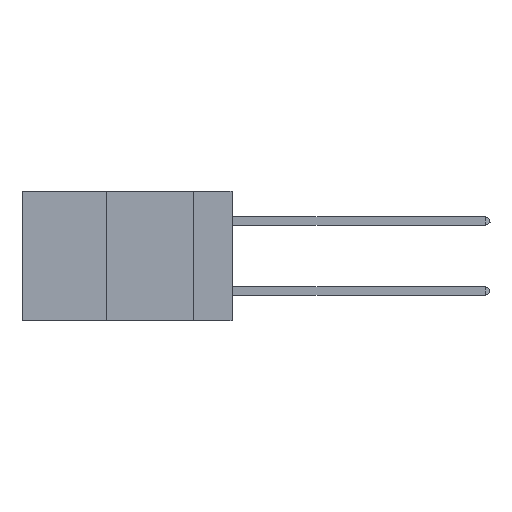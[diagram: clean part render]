
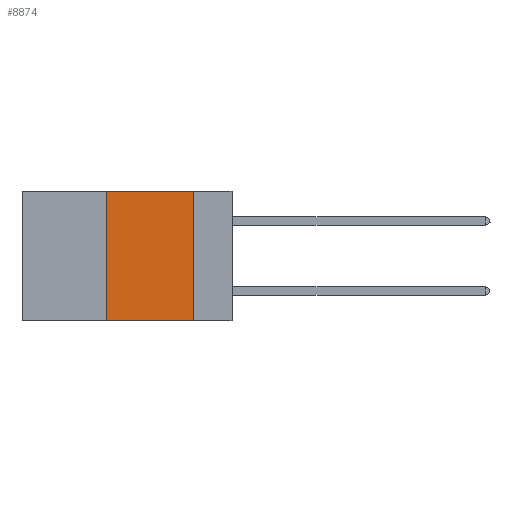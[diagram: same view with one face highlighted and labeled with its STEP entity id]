
A CAD part, left-side view. The second image highlights one B-rep face of the part: STEP entity #8874.
In plain terms, the highlighted planar face has unit normal (-1, 0, 0).
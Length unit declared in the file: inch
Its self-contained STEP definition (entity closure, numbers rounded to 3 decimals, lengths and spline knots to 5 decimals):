
#141 = CARTESIAN_POINT ( 'NONE',  ( 0., 0.36, 0. ) ) ;
#306 = EDGE_CURVE ( 'NONE', #5721, #7778, #2597, .T. ) ;
#1040 = CARTESIAN_POINT ( 'NONE',  ( 0., 0.36, 0. ) ) ;
#1139 = VECTOR ( 'NONE', #14552, 39.37008 ) ;
#1510 = DIRECTION ( 'NONE',  ( 0., 0., 1. ) ) ;
#1676 = VERTEX_POINT ( 'NONE', #1040 ) ;
#2479 = CARTESIAN_POINT ( 'NONE',  ( 0., 0.6, 0. ) ) ;
#2597 = LINE ( 'NONE', #9720, #15960 ) ;
#2968 = LINE ( 'NONE', #141, #13832 ) ;
#3928 = PLANE ( 'NONE',  #8300 ) ;
#4286 = EDGE_CURVE ( 'NONE', #5032, #7778, #17821, .T. ) ;
#4310 = LINE ( 'NONE', #4487, #1139 ) ;
#4471 = ORIENTED_EDGE ( 'NONE', *, *, #4286, .T. ) ;
#4487 = CARTESIAN_POINT ( 'NONE',  ( 0., 0.6, 0. ) ) ;
#5032 = VERTEX_POINT ( 'NONE', #5752 ) ;
#5529 = ORIENTED_EDGE ( 'NONE', *, *, #6562, .F. ) ;
#5721 = VERTEX_POINT ( 'NONE', #11022 ) ;
#5752 = CARTESIAN_POINT ( 'NONE',  ( 0., 0.36, -0.37 ) ) ;
#6289 = VECTOR ( 'NONE', #13340, 39.37008 ) ;
#6562 = EDGE_CURVE ( 'NONE', #5032, #1676, #2968, .T. ) ;
#7778 = VERTEX_POINT ( 'NONE', #13922 ) ;
#8300 = AXIS2_PLACEMENT_3D ( 'NONE', #2479, #8414, #14358 ) ;
#8414 = DIRECTION ( 'NONE',  ( 1., 0., 0. ) ) ;
#8859 = CARTESIAN_POINT ( 'NONE',  ( 0., 0.6, -0.37 ) ) ;
#8874 = ADVANCED_FACE ( 'NONE', ( #12880 ), #3928, .F. ) ;
#9508 = ORIENTED_EDGE ( 'NONE', *, *, #10252, .F. ) ;
#9720 = CARTESIAN_POINT ( 'NONE',  ( 0., 0.11, 0. ) ) ;
#10016 = DIRECTION ( 'NONE',  ( 0., 0., -1. ) ) ;
#10252 = EDGE_CURVE ( 'NONE', #1676, #5721, #4310, .T. ) ;
#11022 = CARTESIAN_POINT ( 'NONE',  ( 0., 0.11, 0. ) ) ;
#12880 = FACE_OUTER_BOUND ( 'NONE', #15478, .T. ) ;
#13340 = DIRECTION ( 'NONE',  ( 0., -1., 0. ) ) ;
#13832 = VECTOR ( 'NONE', #1510, 39.37008 ) ;
#13922 = CARTESIAN_POINT ( 'NONE',  ( 0., 0.11, -0.37 ) ) ;
#14358 = DIRECTION ( 'NONE',  ( 0., 0., -1. ) ) ;
#14552 = DIRECTION ( 'NONE',  ( 0., -1., 0. ) ) ;
#15478 = EDGE_LOOP ( 'NONE', ( #17526, #9508, #5529, #4471 ) ) ;
#15960 = VECTOR ( 'NONE', #10016, 39.37008 ) ;
#17526 = ORIENTED_EDGE ( 'NONE', *, *, #306, .F. ) ;
#17821 = LINE ( 'NONE', #8859, #6289 ) ;
